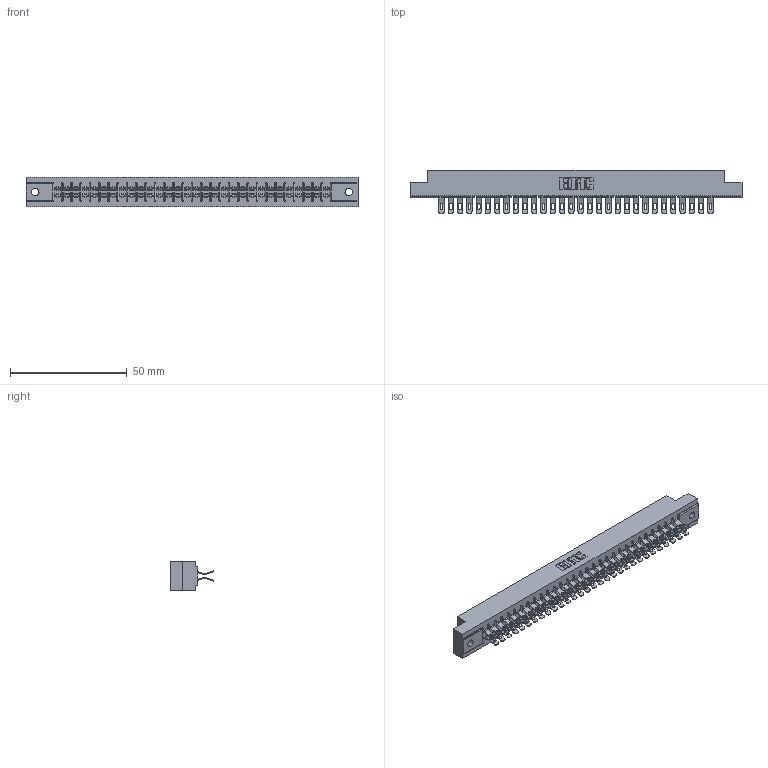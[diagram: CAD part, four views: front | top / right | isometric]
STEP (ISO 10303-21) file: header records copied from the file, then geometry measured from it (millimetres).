
FILE_DESCRIPTION (( 'STEP AP203' ), '1' );
FILE_NAME ('355-060-555-202.STEP', '2019-09-12T13:57:13', ( '' ), ( '' ), 'SwSTEP 2.0', 'SolidWorks 2016', '' );
FILE_SCHEMA (( 'CONFIG_CONTROL_DESIGN' ));
Length unit declared in the file: inch
Products named in the file (3): 305-290-001_555; 355-060-555-202; 305 Part_.128 Dia
Assembly tree (61 placements, depth 2):
  355-060-555-202
    305 Part_.128 Dia
    305-290-001_555  x60
Bounding box: 141.88 x 18.41 x 12.7 mm (x, y, z)
Volume: 14866.2 mm3; surface area: 19504.5 mm2
Topology: 61 solids, 61 shells, 4076 faces, 12166 edges, 7948 vertices
Faces by surface type: plane 1988, cylinder 1968, sphere 120
Entity records: 34569 total; most frequent: CARTESIAN_POINT 5738, ORIENTED_EDGE 5684, DIRECTION 5554, EDGE_CURVE 2842, LINE 2266, VECTOR 2266, VERTEX_POINT 1812, AXIS2_PLACEMENT_3D 1644
